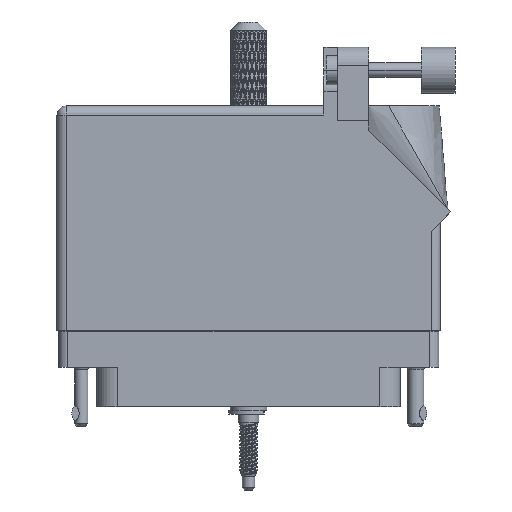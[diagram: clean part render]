
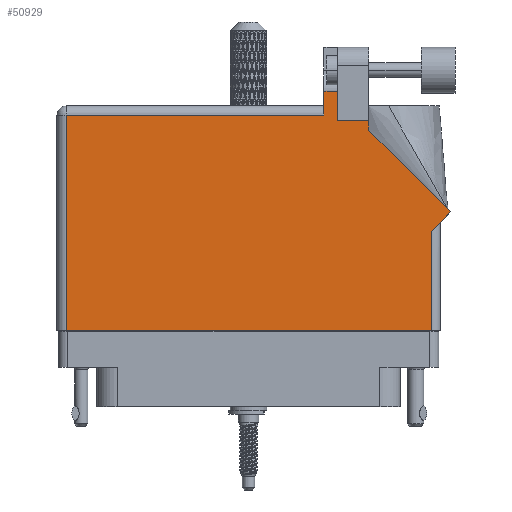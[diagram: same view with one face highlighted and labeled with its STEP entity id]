
A CAD part, front view. The second image highlights one B-rep face of the part: STEP entity #50929.
In plain terms, the highlighted face is planar.
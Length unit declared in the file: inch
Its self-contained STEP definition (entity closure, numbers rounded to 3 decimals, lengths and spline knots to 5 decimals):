
#1170 = VECTOR ( 'NONE', #72362, 39.37008 ) ;
#4460 = CARTESIAN_POINT ( 'NONE',  ( 0.607, 1.33, 0.455 ) ) ;
#6499 = LINE ( 'NONE', #97622, #28887 ) ;
#7890 = ORIENTED_EDGE ( 'NONE', *, *, #57574, .T. ) ;
#9029 = LINE ( 'NONE', #16176, #103880 ) ;
#10018 = VECTOR ( 'NONE', #110118, 39.37008 ) ;
#12479 = VERTEX_POINT ( 'NONE', #103011 ) ;
#14128 = DIRECTION ( 'NONE',  ( 0., -1., 0. ) ) ;
#15260 = ORIENTED_EDGE ( 'NONE', *, *, #121341, .T. ) ;
#16176 = CARTESIAN_POINT ( 'NONE',  ( -1.306, -0.1, 0.455 ) ) ;
#17243 = CARTESIAN_POINT ( 'NONE',  ( -1.306, 1.368, 0.455 ) ) ;
#18281 = LINE ( 'NONE', #104335, #77539 ) ;
#18933 = VERTEX_POINT ( 'NONE', #4460 ) ;
#20709 = LINE ( 'NONE', #106383, #84334 ) ;
#21717 = CARTESIAN_POINT ( 'NONE',  ( 0.82, 1.33, 0.455 ) ) ;
#23546 = EDGE_CURVE ( 'NONE', #94289, #89464, #46067, .T. ) ;
#24393 = CARTESIAN_POINT ( 'NONE',  ( 1.244, 0.637, 0.455 ) ) ;
#25309 = VERTEX_POINT ( 'NONE', #118823 ) ;
#28887 = VECTOR ( 'NONE', #67480, 39.37008 ) ;
#29205 = CARTESIAN_POINT ( 'NONE',  ( 1.244, 0.575, 0.455 ) ) ;
#31040 = ORIENTED_EDGE ( 'NONE', *, *, #76009, .T. ) ;
#34295 = ORIENTED_EDGE ( 'NONE', *, *, #59841, .T. ) ;
#34333 = ORIENTED_EDGE ( 'NONE', *, *, #110929, .T. ) ;
#40688 = DIRECTION ( 'NONE',  ( -1., 0., 0. ) ) ;
#41077 = PLANE ( 'NONE',  #99389 ) ;
#44524 = LINE ( 'NONE', #68545, #114049 ) ;
#44718 = VECTOR ( 'NONE', #87887, 39.37008 ) ;
#46067 = LINE ( 'NONE', #98169, #88972 ) ;
#47619 = CARTESIAN_POINT ( 'NONE',  ( -1.244, -0.1, 0.455 ) ) ;
#50929 = ADVANCED_FACE ( 'NONE', ( #95868 ), #41077, .F. ) ;
#53217 = ORIENTED_EDGE ( 'NONE', *, *, #63209, .T. ) ;
#53397 = ORIENTED_EDGE ( 'NONE', *, *, #23546, .T. ) ;
#57574 = EDGE_CURVE ( 'NONE', #89464, #25309, #9029, .T. ) ;
#58881 = CARTESIAN_POINT ( 'NONE',  ( -1.306, 1.43, 0.455 ) ) ;
#59841 = EDGE_CURVE ( 'NONE', #25309, #101035, #84145, .T. ) ;
#60242 = EDGE_LOOP ( 'NONE', ( #34333, #53217, #31040, #73327, #53397, #7890, #34295, #15260, #80185, #106439, #82749 ) ) ;
#63209 = EDGE_CURVE ( 'NONE', #114680, #89517, #6499, .T. ) ;
#66631 = CARTESIAN_POINT ( 'NONE',  ( 0.513, 1.5315, 0.455 ) ) ;
#67480 = DIRECTION ( 'NONE',  ( -1., 0., 0. ) ) ;
#68545 = CARTESIAN_POINT ( 'NONE',  ( 0.513, 1.43, 0.455 ) ) ;
#70132 = VECTOR ( 'NONE', #111162, 39.37008 ) ;
#70317 = CARTESIAN_POINT ( 'NONE',  ( 0.607, 1.5315, 0.455 ) ) ;
#72182 = CARTESIAN_POINT ( 'NONE',  ( 0.82, 1.26442, 0.455 ) ) ;
#72362 = DIRECTION ( 'NONE',  ( 0., 1., 0. ) ) ;
#73244 = EDGE_CURVE ( 'NONE', #119256, #94289, #107159, .T. ) ;
#73327 = ORIENTED_EDGE ( 'NONE', *, *, #73244, .T. ) ;
#74583 = CARTESIAN_POINT ( 'NONE',  ( 0.82, 1.26442, 0.455 ) ) ;
#76009 = EDGE_CURVE ( 'NONE', #89517, #119256, #44524, .T. ) ;
#77539 = VECTOR ( 'NONE', #114617, 39.37008 ) ;
#78062 = LINE ( 'NONE', #74583, #112082 ) ;
#79131 = CARTESIAN_POINT ( 'NONE',  ( 1.37671, 0.70771, 0.455 ) ) ;
#80185 = ORIENTED_EDGE ( 'NONE', *, *, #83345, .T. ) ;
#82427 = DIRECTION ( 'NONE',  ( 1., 0., 0. ) ) ;
#82749 = ORIENTED_EDGE ( 'NONE', *, *, #96499, .T. ) ;
#83345 = EDGE_CURVE ( 'NONE', #106589, #87736, #20709, .T. ) ;
#84145 = LINE ( 'NONE', #24393, #1170 ) ;
#84334 = VECTOR ( 'NONE', #115908, 39.37008 ) ;
#87736 = VERTEX_POINT ( 'NONE', #72182 ) ;
#87887 = DIRECTION ( 'NONE',  ( -1., 0., 0. ) ) ;
#88972 = VECTOR ( 'NONE', #14128, 39.37008 ) ;
#89464 = VERTEX_POINT ( 'NONE', #47619 ) ;
#89517 = VERTEX_POINT ( 'NONE', #66631 ) ;
#94289 = VERTEX_POINT ( 'NONE', #115313 ) ;
#95868 = FACE_OUTER_BOUND ( 'NONE', #60242, .T. ) ;
#96499 = EDGE_CURVE ( 'NONE', #12479, #18933, #114228, .T. ) ;
#97324 = DIRECTION ( 'NONE',  ( 0., 0., -1. ) ) ;
#97486 = LINE ( 'NONE', #120451, #10018 ) ;
#97622 = CARTESIAN_POINT ( 'NONE',  ( 0.93777, 1.5315, 0.455 ) ) ;
#98169 = CARTESIAN_POINT ( 'NONE',  ( -1.244, -0.1, 0.455 ) ) ;
#99389 = AXIS2_PLACEMENT_3D ( 'NONE', #58881, #97324, #40688 ) ;
#101035 = VERTEX_POINT ( 'NONE', #29205 ) ;
#103011 = CARTESIAN_POINT ( 'NONE',  ( 0.82, 1.33, 0.455 ) ) ;
#103880 = VECTOR ( 'NONE', #82427, 39.37008 ) ;
#104335 = CARTESIAN_POINT ( 'NONE',  ( 1.306, 0.637, 0.455 ) ) ;
#105054 = CARTESIAN_POINT ( 'NONE',  ( 0.513, 1.368, 0.455 ) ) ;
#105791 = DIRECTION ( 'NONE',  ( 0., -1., 0. ) ) ;
#106383 = CARTESIAN_POINT ( 'NONE',  ( 1.37671, 0.70771, 0.455 ) ) ;
#106439 = ORIENTED_EDGE ( 'NONE', *, *, #113450, .T. ) ;
#106589 = VERTEX_POINT ( 'NONE', #79131 ) ;
#107159 = LINE ( 'NONE', #17243, #70132 ) ;
#110118 = DIRECTION ( 'NONE',  ( 0., 1., 0. ) ) ;
#110929 = EDGE_CURVE ( 'NONE', #18933, #114680, #97486, .T. ) ;
#110993 = DIRECTION ( 'NONE',  ( 0., 1., 0. ) ) ;
#111162 = DIRECTION ( 'NONE',  ( -1., 0., 0. ) ) ;
#112082 = VECTOR ( 'NONE', #110993, 39.37008 ) ;
#113450 = EDGE_CURVE ( 'NONE', #87736, #12479, #78062, .T. ) ;
#114049 = VECTOR ( 'NONE', #105791, 39.37008 ) ;
#114228 = LINE ( 'NONE', #21717, #44718 ) ;
#114617 = DIRECTION ( 'NONE',  ( 0.707, 0.707, 0. ) ) ;
#114680 = VERTEX_POINT ( 'NONE', #70317 ) ;
#115313 = CARTESIAN_POINT ( 'NONE',  ( -1.244, 1.368, 0.455 ) ) ;
#115908 = DIRECTION ( 'NONE',  ( -0.707, 0.707, 0. ) ) ;
#118823 = CARTESIAN_POINT ( 'NONE',  ( 1.244, -0.1, 0.455 ) ) ;
#119256 = VERTEX_POINT ( 'NONE', #105054 ) ;
#120451 = CARTESIAN_POINT ( 'NONE',  ( 0.607, 1.33, 0.455 ) ) ;
#121341 = EDGE_CURVE ( 'NONE', #101035, #106589, #18281, .T. ) ;
